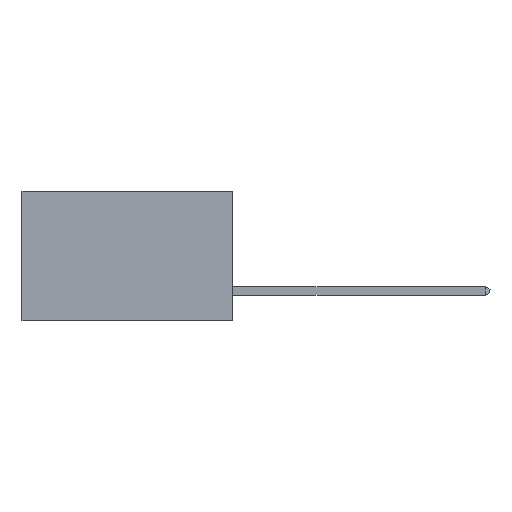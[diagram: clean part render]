
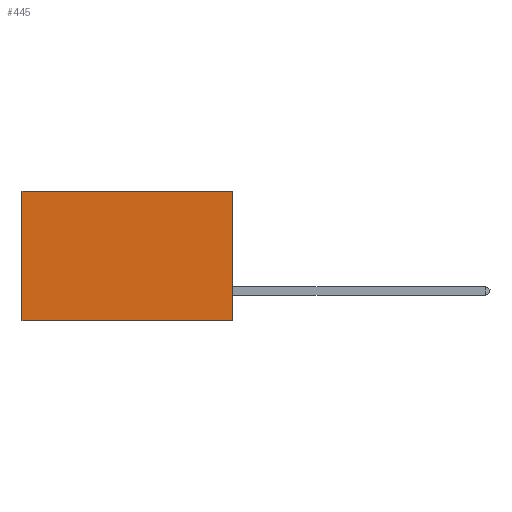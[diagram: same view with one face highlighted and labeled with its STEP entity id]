
A CAD part, left-side view. The second image highlights one B-rep face of the part: STEP entity #445.
In plain terms, the highlighted planar face has unit normal (-1, 0, 0).
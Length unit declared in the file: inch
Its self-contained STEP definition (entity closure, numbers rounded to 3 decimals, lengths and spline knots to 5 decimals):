
#416 = VERTEX_POINT ( 'NONE', #4445 ) ;
#445 = ADVANCED_FACE ( 'NONE', ( #11648 ), #3201, .F. ) ;
#1063 = VERTEX_POINT ( 'NONE', #8303 ) ;
#1450 = ORIENTED_EDGE ( 'NONE', *, *, #8314, .T. ) ;
#1704 = LINE ( 'NONE', #8165, #3722 ) ;
#1725 = CARTESIAN_POINT ( 'NONE',  ( 0.2875, 0., -0.37 ) ) ;
#1992 = ORIENTED_EDGE ( 'NONE', *, *, #7918, .F. ) ;
#2084 = DIRECTION ( 'NONE',  ( 1., 0., 0. ) ) ;
#2263 = LINE ( 'NONE', #7769, #7983 ) ;
#2339 = VECTOR ( 'NONE', #2521, 39.37008 ) ;
#2398 = ORIENTED_EDGE ( 'NONE', *, *, #4863, .T. ) ;
#2521 = DIRECTION ( 'NONE',  ( 0., 0., -1. ) ) ;
#3201 = PLANE ( 'NONE',  #8053 ) ;
#3465 = LINE ( 'NONE', #1725, #15293 ) ;
#3500 = VERTEX_POINT ( 'NONE', #11842 ) ;
#3722 = VECTOR ( 'NONE', #10709, 39.37008 ) ;
#4445 = CARTESIAN_POINT ( 'NONE',  ( 0.2875, 0., 0. ) ) ;
#4863 = EDGE_CURVE ( 'NONE', #3500, #1063, #13228, .T. ) ;
#6620 = DIRECTION ( 'NONE',  ( 0., 0., -1. ) ) ;
#7309 = CARTESIAN_POINT ( 'NONE',  ( 0.2875, 0., -0.37 ) ) ;
#7570 = DIRECTION ( 'NONE',  ( 0., 0., -1. ) ) ;
#7769 = CARTESIAN_POINT ( 'NONE',  ( 0.2875, 0., 0. ) ) ;
#7918 = EDGE_CURVE ( 'NONE', #416, #14338, #2263, .T. ) ;
#7983 = VECTOR ( 'NONE', #7570, 39.37008 ) ;
#8053 = AXIS2_PLACEMENT_3D ( 'NONE', #11426, #2084, #6620 ) ;
#8165 = CARTESIAN_POINT ( 'NONE',  ( 0.2875, 0., 0. ) ) ;
#8303 = CARTESIAN_POINT ( 'NONE',  ( 0.2875, 0.6, -0.37 ) ) ;
#8314 = EDGE_CURVE ( 'NONE', #416, #3500, #1704, .T. ) ;
#10176 = EDGE_CURVE ( 'NONE', #14338, #1063, #3465, .T. ) ;
#10709 = DIRECTION ( 'NONE',  ( 0., 1., 0. ) ) ;
#11134 = EDGE_LOOP ( 'NONE', ( #2398, #11575, #1992, #1450 ) ) ;
#11426 = CARTESIAN_POINT ( 'NONE',  ( 0.2875, 0., 0. ) ) ;
#11575 = ORIENTED_EDGE ( 'NONE', *, *, #10176, .F. ) ;
#11648 = FACE_OUTER_BOUND ( 'NONE', #11134, .T. ) ;
#11842 = CARTESIAN_POINT ( 'NONE',  ( 0.2875, 0.6, 0. ) ) ;
#13228 = LINE ( 'NONE', #14248, #2339 ) ;
#13374 = DIRECTION ( 'NONE',  ( 0., 1., 0. ) ) ;
#14248 = CARTESIAN_POINT ( 'NONE',  ( 0.2875, 0.6, 0. ) ) ;
#14338 = VERTEX_POINT ( 'NONE', #7309 ) ;
#15293 = VECTOR ( 'NONE', #13374, 39.37008 ) ;
